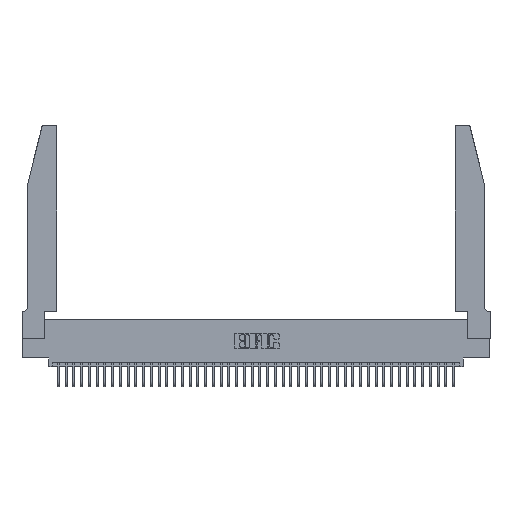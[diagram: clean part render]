
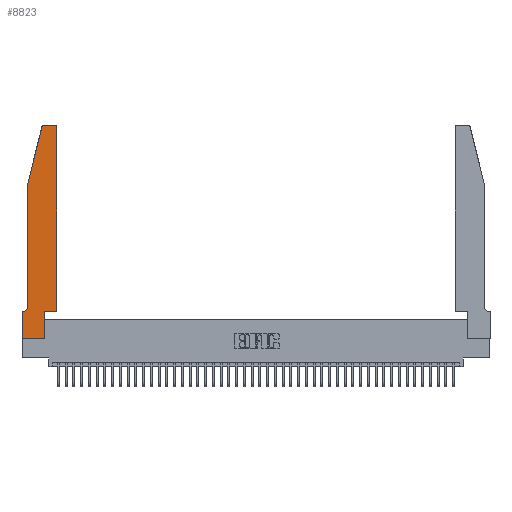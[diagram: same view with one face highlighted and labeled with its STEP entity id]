
A CAD part, top view. The second image highlights one B-rep face of the part: STEP entity #8823.
In plain terms, the highlighted planar face has unit normal (0, 0, 1).
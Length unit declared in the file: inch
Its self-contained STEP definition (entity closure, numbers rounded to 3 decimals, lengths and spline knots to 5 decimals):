
#56 = VECTOR ( 'NONE', #28427, 39.37008 ) ;
#1009 = LINE ( 'NONE', #12940, #8749 ) ;
#1142 = CARTESIAN_POINT ( 'NONE',  ( 0.4205, 2.72, 0.37 ) ) ;
#2272 = CARTESIAN_POINT ( 'NONE',  ( 0.2605, 2.75, 0.37 ) ) ;
#2444 = CARTESIAN_POINT ( 'NONE',  ( 0.4505, 0.35, 0.37 ) ) ;
#2475 = EDGE_CURVE ( 'NONE', #33205, #25564, #1009, .T. ) ;
#2917 = AXIS2_PLACEMENT_3D ( 'NONE', #1142, #24167, #4478 ) ;
#3036 = DIRECTION ( 'NONE',  ( 0., 0., -1. ) ) ;
#3616 = CARTESIAN_POINT ( 'NONE',  ( 0.0055, 0.35, 0.37 ) ) ;
#4478 = DIRECTION ( 'NONE',  ( 1., 0., 0. ) ) ;
#5525 = ORIENTED_EDGE ( 'NONE', *, *, #22855, .T. ) ;
#5781 = DIRECTION ( 'NONE',  ( -0.239, -0.971, 0. ) ) ;
#5855 = AXIS2_PLACEMENT_3D ( 'NONE', #22717, #3036, #26098 ) ;
#6069 = DIRECTION ( 'NONE',  ( 1., 0., 0. ) ) ;
#6451 = EDGE_CURVE ( 'NONE', #25564, #11378, #15990, .T. ) ;
#6823 = CARTESIAN_POINT ( 'NONE',  ( 0.4205, 2.75, 0.37 ) ) ;
#6933 = EDGE_CURVE ( 'NONE', #28348, #16608, #32452, .T. ) ;
#8749 = VECTOR ( 'NONE', #19548, 39.37008 ) ;
#8823 = ADVANCED_FACE ( 'NONE', ( #33282 ), #9903, .T. ) ;
#8901 = DIRECTION ( 'NONE',  ( -1., 0., 0. ) ) ;
#8935 = VECTOR ( 'NONE', #6069, 39.37008 ) ;
#9057 = DIRECTION ( 'NONE',  ( 1., 0., 0. ) ) ;
#9266 = DIRECTION ( 'NONE',  ( 0., 0., 1. ) ) ;
#9479 = LINE ( 'NONE', #18824, #25979 ) ;
#9903 = PLANE ( 'NONE',  #19916 ) ;
#10047 = EDGE_CURVE ( 'NONE', #28962, #41230, #35237, .T. ) ;
#11328 = ORIENTED_EDGE ( 'NONE', *, *, #38767, .T. ) ;
#11378 = VERTEX_POINT ( 'NONE', #3616 ) ;
#11411 = AXIS2_PLACEMENT_3D ( 'NONE', #29016, #9266, #32326 ) ;
#11532 = CARTESIAN_POINT ( 'NONE',  ( 0.4505, 0.35, 0.37 ) ) ;
#12408 = EDGE_CURVE ( 'NONE', #16608, #15840, #36250, .T. ) ;
#12940 = CARTESIAN_POINT ( 'NONE',  ( 0.0755, 2., 0.37 ) ) ;
#13458 = CARTESIAN_POINT ( 'NONE',  ( 0.4505, 0.35, 0.37 ) ) ;
#14052 = VERTEX_POINT ( 'NONE', #40605 ) ;
#15086 = ORIENTED_EDGE ( 'NONE', *, *, #6933, .T. ) ;
#15840 = VERTEX_POINT ( 'NONE', #24879 ) ;
#15945 = ORIENTED_EDGE ( 'NONE', *, *, #29858, .T. ) ;
#15990 = CIRCLE ( 'NONE', #5855, 0.07 ) ;
#16453 = ORIENTED_EDGE ( 'NONE', *, *, #10047, .T. ) ;
#16608 = VERTEX_POINT ( 'NONE', #39307 ) ;
#18824 = CARTESIAN_POINT ( 'NONE',  ( 0.0755, 2., 0.37 ) ) ;
#19548 = DIRECTION ( 'NONE',  ( 0., -1., 0. ) ) ;
#19788 = DIRECTION ( 'NONE',  ( 1., 0., 0. ) ) ;
#19916 = AXIS2_PLACEMENT_3D ( 'NONE', #22944, #39611, #19788 ) ;
#21376 = VERTEX_POINT ( 'NONE', #37107 ) ;
#21494 = VERTEX_POINT ( 'NONE', #37686 ) ;
#21768 = CARTESIAN_POINT ( 'NONE',  ( 0.2865, 0.35, 0.37 ) ) ;
#22099 = EDGE_CURVE ( 'NONE', #15840, #33205, #9479, .T. ) ;
#22717 = CARTESIAN_POINT ( 'NONE',  ( 0.0055, 0.42, 0.37 ) ) ;
#22855 = EDGE_CURVE ( 'NONE', #26644, #21494, #23281, .T. ) ;
#22944 = CARTESIAN_POINT ( 'NONE',  ( 0., 0.35, 0.37 ) ) ;
#23057 = VECTOR ( 'NONE', #25114, 39.37008 ) ;
#23281 = LINE ( 'NONE', #11532, #39876 ) ;
#23643 = VECTOR ( 'NONE', #8901, 39.37008 ) ;
#24167 = DIRECTION ( 'NONE',  ( 0., 0., 1. ) ) ;
#24379 = VECTOR ( 'NONE', #9057, 39.37008 ) ;
#24777 = CARTESIAN_POINT ( 'NONE',  ( 0.0755, 0.42, 0.37 ) ) ;
#24879 = CARTESIAN_POINT ( 'NONE',  ( 0.25487, 2.72718, 0.37 ) ) ;
#25114 = DIRECTION ( 'NONE',  ( 0., 1., 0. ) ) ;
#25214 = CARTESIAN_POINT ( 'NONE',  ( 0.0755, 0.35, 0.37 ) ) ;
#25425 = LINE ( 'NONE', #2444, #24379 ) ;
#25564 = VERTEX_POINT ( 'NONE', #24777 ) ;
#25979 = VECTOR ( 'NONE', #5781, 39.37008 ) ;
#26094 = CARTESIAN_POINT ( 'NONE',  ( 0., 0., 0.37 ) ) ;
#26098 = DIRECTION ( 'NONE',  ( -1., 0., 0. ) ) ;
#26440 = CIRCLE ( 'NONE', #2917, 0.03 ) ;
#26644 = VERTEX_POINT ( 'NONE', #13458 ) ;
#26789 = ORIENTED_EDGE ( 'NONE', *, *, #12408, .T. ) ;
#26858 = CARTESIAN_POINT ( 'NONE',  ( 0.2865, 0., 0.37 ) ) ;
#26978 = ORIENTED_EDGE ( 'NONE', *, *, #27525, .T. ) ;
#27525 = EDGE_CURVE ( 'NONE', #11378, #21376, #28448, .T. ) ;
#27981 = CARTESIAN_POINT ( 'NONE',  ( 0.0755, 2., 0.37 ) ) ;
#28348 = VERTEX_POINT ( 'NONE', #6823 ) ;
#28427 = DIRECTION ( 'NONE',  ( -1., 0., 0. ) ) ;
#28439 = ORIENTED_EDGE ( 'NONE', *, *, #33388, .T. ) ;
#28448 = LINE ( 'NONE', #25214, #56 ) ;
#28962 = VERTEX_POINT ( 'NONE', #33116 ) ;
#29016 = CARTESIAN_POINT ( 'NONE',  ( 0.284, 2.72, 0.37 ) ) ;
#29111 = CARTESIAN_POINT ( 'NONE',  ( 0., 0., 0.37 ) ) ;
#29206 = ORIENTED_EDGE ( 'NONE', *, *, #22099, .T. ) ;
#29316 = VECTOR ( 'NONE', #42535, 39.37008 ) ;
#29858 = EDGE_CURVE ( 'NONE', #41230, #14052, #40680, .T. ) ;
#32326 = DIRECTION ( 'NONE',  ( 1., 0., 0. ) ) ;
#32452 = LINE ( 'NONE', #2272, #23643 ) ;
#33116 = CARTESIAN_POINT ( 'NONE',  ( 0., 0., 0.37 ) ) ;
#33205 = VERTEX_POINT ( 'NONE', #27981 ) ;
#33282 = FACE_OUTER_BOUND ( 'NONE', #39839, .T. ) ;
#33388 = EDGE_CURVE ( 'NONE', #14052, #26644, #25425, .T. ) ;
#35237 = LINE ( 'NONE', #29111, #8935 ) ;
#35504 = ORIENTED_EDGE ( 'NONE', *, *, #6451, .T. ) ;
#36250 = CIRCLE ( 'NONE', #11411, 0.03 ) ;
#36621 = EDGE_CURVE ( 'NONE', #21494, #28348, #26440, .T. ) ;
#37107 = CARTESIAN_POINT ( 'NONE',  ( 0., 0.35, 0.37 ) ) ;
#37686 = CARTESIAN_POINT ( 'NONE',  ( 0.4505, 2.72, 0.37 ) ) ;
#38096 = LINE ( 'NONE', #26094, #29316 ) ;
#38333 = ORIENTED_EDGE ( 'NONE', *, *, #2475, .T. ) ;
#38380 = ORIENTED_EDGE ( 'NONE', *, *, #36621, .T. ) ;
#38767 = EDGE_CURVE ( 'NONE', #21376, #28962, #38096, .T. ) ;
#39307 = CARTESIAN_POINT ( 'NONE',  ( 0.284, 2.75, 0.37 ) ) ;
#39611 = DIRECTION ( 'NONE',  ( 0., 0., 1. ) ) ;
#39839 = EDGE_LOOP ( 'NONE', ( #15086, #26789, #29206, #38333, #35504, #26978, #11328, #16453, #15945, #28439, #5525, #38380 ) ) ;
#39876 = VECTOR ( 'NONE', #41399, 39.37008 ) ;
#40605 = CARTESIAN_POINT ( 'NONE',  ( 0.2865, 0.35, 0.37 ) ) ;
#40680 = LINE ( 'NONE', #21768, #23057 ) ;
#41230 = VERTEX_POINT ( 'NONE', #26858 ) ;
#41399 = DIRECTION ( 'NONE',  ( 0., 1., 0. ) ) ;
#42535 = DIRECTION ( 'NONE',  ( 0., -1., 0. ) ) ;
